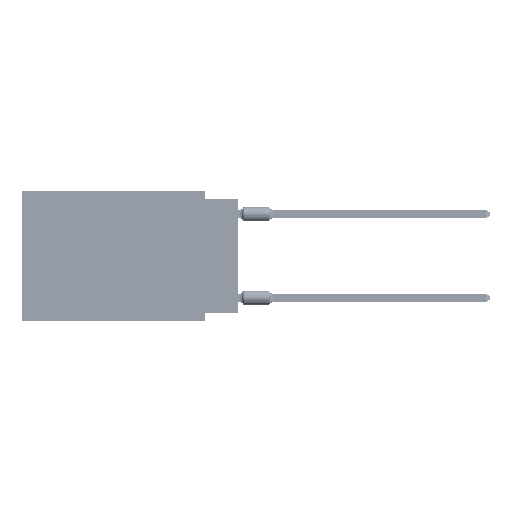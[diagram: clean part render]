
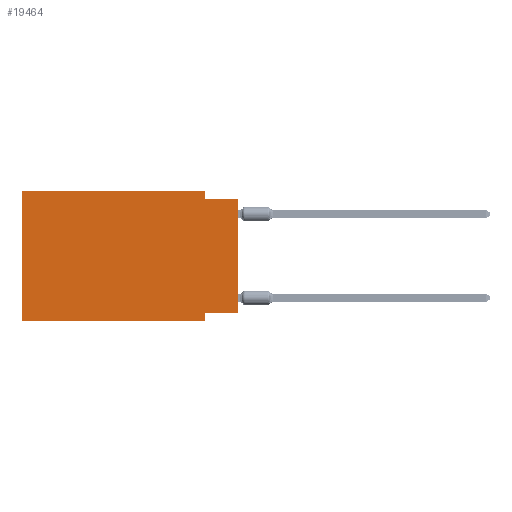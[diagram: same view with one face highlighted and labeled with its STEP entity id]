
A CAD part, left-side view. The second image highlights one B-rep face of the part: STEP entity #19464.
In plain terms, the highlighted planar face has unit normal (-1, 0, 0).
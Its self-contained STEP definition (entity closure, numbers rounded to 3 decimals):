
#1277 = EDGE_CURVE ( 'NONE', #71546, #34832, #23700, .T. ) ;
#2319 = VERTEX_POINT ( 'NONE', #19311 ) ;
#3072 = VERTEX_POINT ( 'NONE', #3780 ) ;
#3248 = FACE_OUTER_BOUND ( 'NONE', #47139, .T. ) ;
#3780 = CARTESIAN_POINT ( 'NONE',  ( 0., 2.54, 0. ) ) ;
#4789 = VECTOR ( 'NONE', #16673, 1000. ) ;
#4953 = VERTEX_POINT ( 'NONE', #38899 ) ;
#5129 = EDGE_CURVE ( 'NONE', #71546, #2319, #46875, .T. ) ;
#5758 = ORIENTED_EDGE ( 'NONE', *, *, #38202, .F. ) ;
#7250 = ORIENTED_EDGE ( 'NONE', *, *, #34468, .F. ) ;
#7372 = VECTOR ( 'NONE', #31777, 1000. ) ;
#7521 = ORIENTED_EDGE ( 'NONE', *, *, #67069, .F. ) ;
#8124 = CARTESIAN_POINT ( 'NONE',  ( 0., 2.54, -9.906 ) ) ;
#9612 = LINE ( 'NONE', #43392, #7372 ) ;
#13001 = VECTOR ( 'NONE', #14487, 1000. ) ;
#14463 = CARTESIAN_POINT ( 'NONE',  ( 0., 2.54, 0. ) ) ;
#14487 = DIRECTION ( 'NONE',  ( 0., -1., 0. ) ) ;
#14866 = CARTESIAN_POINT ( 'NONE',  ( 0., 16.383, 0. ) ) ;
#16514 = EDGE_CURVE ( 'NONE', #2319, #38760, #9612, .T. ) ;
#16673 = DIRECTION ( 'NONE',  ( 0., 0., 1. ) ) ;
#18121 = VERTEX_POINT ( 'NONE', #46126 ) ;
#19311 = CARTESIAN_POINT ( 'NONE',  ( 0., 2.54, -9.271 ) ) ;
#19464 = ADVANCED_FACE ( 'NONE', ( #3248 ), #19950, .F. ) ;
#19553 = CARTESIAN_POINT ( 'NONE',  ( 0., 16.383, -9.906 ) ) ;
#19950 = PLANE ( 'NONE',  #60958 ) ;
#22523 = VECTOR ( 'NONE', #39347, 1000. ) ;
#23700 = LINE ( 'NONE', #34602, #22523 ) ;
#25172 = ORIENTED_EDGE ( 'NONE', *, *, #16514, .F. ) ;
#28515 = CARTESIAN_POINT ( 'NONE',  ( 0., 0., -0.635 ) ) ;
#29758 = CARTESIAN_POINT ( 'NONE',  ( 0., 0., -9.271 ) ) ;
#31195 = CARTESIAN_POINT ( 'NONE',  ( 0., 16.383, 0. ) ) ;
#31777 = DIRECTION ( 'NONE',  ( 0., 0., -1. ) ) ;
#34157 = CARTESIAN_POINT ( 'NONE',  ( 0., 0., -9.271 ) ) ;
#34468 = EDGE_CURVE ( 'NONE', #69825, #34832, #53983, .T. ) ;
#34602 = CARTESIAN_POINT ( 'NONE',  ( 0., 0., 0. ) ) ;
#34832 = VERTEX_POINT ( 'NONE', #28515 ) ;
#38202 = EDGE_CURVE ( 'NONE', #4953, #18121, #39199, .T. ) ;
#38446 = EDGE_CURVE ( 'NONE', #4953, #38760, #56977, .T. ) ;
#38760 = VERTEX_POINT ( 'NONE', #8124 ) ;
#38899 = CARTESIAN_POINT ( 'NONE',  ( 0., 16.383, -9.906 ) ) ;
#39199 = LINE ( 'NONE', #66790, #4789 ) ;
#39347 = DIRECTION ( 'NONE',  ( 0., 0., 1. ) ) ;
#39440 = ORIENTED_EDGE ( 'NONE', *, *, #38446, .T. ) ;
#41720 = DIRECTION ( 'NONE',  ( 0., -1., 0. ) ) ;
#43392 = CARTESIAN_POINT ( 'NONE',  ( 0., 2.54, -9.906 ) ) ;
#44919 = VECTOR ( 'NONE', #69027, 1000. ) ;
#45439 = VECTOR ( 'NONE', #41720, 1000. ) ;
#45942 = VECTOR ( 'NONE', #52920, 1000. ) ;
#46126 = CARTESIAN_POINT ( 'NONE',  ( 0., 16.383, 0. ) ) ;
#46875 = LINE ( 'NONE', #34157, #44919 ) ;
#46902 = ORIENTED_EDGE ( 'NONE', *, *, #56280, .F. ) ;
#47139 = EDGE_LOOP ( 'NONE', ( #67951, #7250, #7521, #46902, #5758, #39440, #25172, #71182 ) ) ;
#47914 = LINE ( 'NONE', #31195, #13001 ) ;
#52920 = DIRECTION ( 'NONE',  ( 0., -1., 0. ) ) ;
#52981 = LINE ( 'NONE', #14463, #64426 ) ;
#53387 = DIRECTION ( 'NONE',  ( 0., 0., -1. ) ) ;
#53737 = DIRECTION ( 'NONE',  ( 1., 0., 0. ) ) ;
#53983 = LINE ( 'NONE', #63808, #45942 ) ;
#56280 = EDGE_CURVE ( 'NONE', #18121, #3072, #47914, .T. ) ;
#56977 = LINE ( 'NONE', #19553, #45439 ) ;
#57440 = CARTESIAN_POINT ( 'NONE',  ( 0., 2.54, -0.635 ) ) ;
#60958 = AXIS2_PLACEMENT_3D ( 'NONE', #14866, #53737, #53387 ) ;
#63808 = CARTESIAN_POINT ( 'NONE',  ( 0., 0., -0.635 ) ) ;
#64426 = VECTOR ( 'NONE', #68611, 1000. ) ;
#66790 = CARTESIAN_POINT ( 'NONE',  ( 0., 16.383, 0. ) ) ;
#67069 = EDGE_CURVE ( 'NONE', #3072, #69825, #52981, .T. ) ;
#67951 = ORIENTED_EDGE ( 'NONE', *, *, #1277, .T. ) ;
#68611 = DIRECTION ( 'NONE',  ( 0., 0., -1. ) ) ;
#69027 = DIRECTION ( 'NONE',  ( 0., 1., 0. ) ) ;
#69825 = VERTEX_POINT ( 'NONE', #57440 ) ;
#71182 = ORIENTED_EDGE ( 'NONE', *, *, #5129, .F. ) ;
#71546 = VERTEX_POINT ( 'NONE', #29758 ) ;
